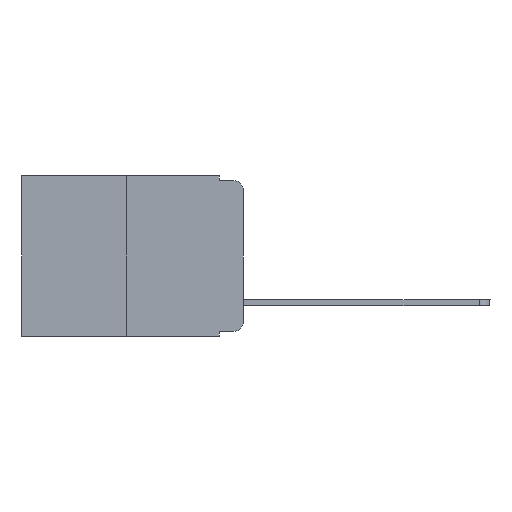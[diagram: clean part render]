
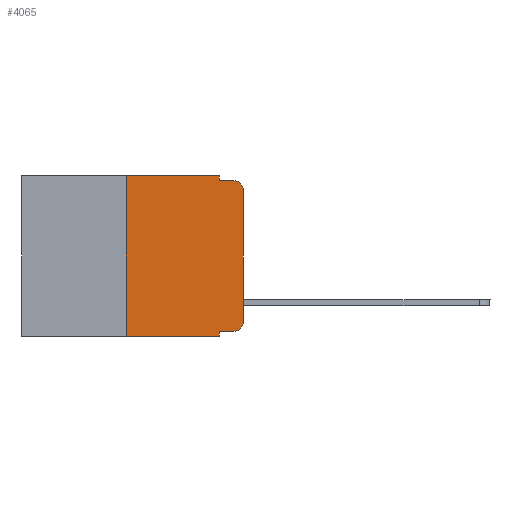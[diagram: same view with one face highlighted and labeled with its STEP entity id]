
A CAD part, left-side view. The second image highlights one B-rep face of the part: STEP entity #4065.
In plain terms, the highlighted planar face has unit normal (-1, 0, 0).
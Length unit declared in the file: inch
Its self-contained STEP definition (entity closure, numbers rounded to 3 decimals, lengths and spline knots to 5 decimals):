
#213 = EDGE_CURVE ( 'NONE', #11336, #13138, #16758, .T. ) ;
#767 = ORIENTED_EDGE ( 'NONE', *, *, #12432, .T. ) ;
#989 = LINE ( 'NONE', #15882, #3333 ) ;
#1069 = EDGE_CURVE ( 'NONE', #6605, #21570, #11862, .T. ) ;
#1149 = ORIENTED_EDGE ( 'NONE', *, *, #22237, .F. ) ;
#1440 = DIRECTION ( 'NONE',  ( 1., 0., 0. ) ) ;
#1817 = EDGE_CURVE ( 'NONE', #21570, #15381, #14677, .T. ) ;
#2532 = CARTESIAN_POINT ( 'NONE',  ( 0., 0.25, 0. ) ) ;
#2564 = VERTEX_POINT ( 'NONE', #3204 ) ;
#2614 = EDGE_CURVE ( 'NONE', #13138, #15381, #2838, .T. ) ;
#2838 = LINE ( 'NONE', #19522, #16950 ) ;
#2845 = DIRECTION ( 'NONE',  ( 0., -1., 0. ) ) ;
#2969 = EDGE_CURVE ( 'NONE', #3411, #2564, #989, .T. ) ;
#3204 = CARTESIAN_POINT ( 'NONE',  ( 0., 0.051, -0.343 ) ) ;
#3275 = CARTESIAN_POINT ( 'NONE',  ( 0., 0., -0.03 ) ) ;
#3333 = VECTOR ( 'NONE', #17605, 39.37008 ) ;
#3411 = VERTEX_POINT ( 'NONE', #10859 ) ;
#3567 = EDGE_LOOP ( 'NONE', ( #13214, #23294, #11967, #9759, #11827, #14202, #8926, #1149, #767, #23444 ) ) ;
#3739 = AXIS2_PLACEMENT_3D ( 'NONE', #19326, #1440, #18484 ) ;
#4037 = EDGE_CURVE ( 'NONE', #23215, #11336, #21836, .T. ) ;
#4065 = ADVANCED_FACE ( 'NONE', ( #21272 ), #13122, .F. ) ;
#5143 = CARTESIAN_POINT ( 'NONE',  ( 0., 0.02, -0.313 ) ) ;
#5422 = VECTOR ( 'NONE', #14570, 39.37008 ) ;
#6605 = VERTEX_POINT ( 'NONE', #20933 ) ;
#6629 = VERTEX_POINT ( 'NONE', #16283 ) ;
#6677 = VECTOR ( 'NONE', #22889, 39.37008 ) ;
#6799 = CARTESIAN_POINT ( 'NONE',  ( 0., 0., 0. ) ) ;
#8610 = AXIS2_PLACEMENT_3D ( 'NONE', #5143, #16107, #12559 ) ;
#8926 = ORIENTED_EDGE ( 'NONE', *, *, #2969, .T. ) ;
#9759 = ORIENTED_EDGE ( 'NONE', *, *, #213, .F. ) ;
#9852 = CIRCLE ( 'NONE', #8610, 0.02 ) ;
#9926 = CARTESIAN_POINT ( 'NONE',  ( 0., 0.051, -0.01 ) ) ;
#10859 = CARTESIAN_POINT ( 'NONE',  ( 0., 0.25, -0.343 ) ) ;
#10968 = LINE ( 'NONE', #19334, #14087 ) ;
#11261 = DIRECTION ( 'NONE',  ( 0., 0., 1. ) ) ;
#11336 = VERTEX_POINT ( 'NONE', #17613 ) ;
#11827 = ORIENTED_EDGE ( 'NONE', *, *, #4037, .F. ) ;
#11862 = LINE ( 'NONE', #6799, #14720 ) ;
#11967 = ORIENTED_EDGE ( 'NONE', *, *, #2614, .F. ) ;
#12007 = VECTOR ( 'NONE', #22891, 39.37008 ) ;
#12027 = CARTESIAN_POINT ( 'NONE',  ( 0., 0.02, -0.03 ) ) ;
#12432 = EDGE_CURVE ( 'NONE', #13806, #6629, #21845, .T. ) ;
#12559 = DIRECTION ( 'NONE',  ( 0., 0., -1. ) ) ;
#12675 = AXIS2_PLACEMENT_3D ( 'NONE', #12027, #14010, #16191 ) ;
#13122 = PLANE ( 'NONE',  #3739 ) ;
#13138 = VERTEX_POINT ( 'NONE', #9926 ) ;
#13214 = ORIENTED_EDGE ( 'NONE', *, *, #1069, .T. ) ;
#13806 = VERTEX_POINT ( 'NONE', #16899 ) ;
#13871 = CARTESIAN_POINT ( 'NONE',  ( 0., 0.473, 0. ) ) ;
#14010 = DIRECTION ( 'NONE',  ( -1., 0., 0. ) ) ;
#14087 = VECTOR ( 'NONE', #11261, 39.37008 ) ;
#14202 = ORIENTED_EDGE ( 'NONE', *, *, #21971, .F. ) ;
#14570 = DIRECTION ( 'NONE',  ( 0., 0., -1. ) ) ;
#14677 = CIRCLE ( 'NONE', #12675, 0.02 ) ;
#14720 = VECTOR ( 'NONE', #21458, 39.37008 ) ;
#15381 = VERTEX_POINT ( 'NONE', #16945 ) ;
#15754 = CARTESIAN_POINT ( 'NONE',  ( 0., 0.051, -0.333 ) ) ;
#15882 = CARTESIAN_POINT ( 'NONE',  ( 0., 0.473, -0.343 ) ) ;
#16107 = DIRECTION ( 'NONE',  ( -1., 0., 0. ) ) ;
#16191 = DIRECTION ( 'NONE',  ( 0., 0., -1. ) ) ;
#16240 = EDGE_CURVE ( 'NONE', #6629, #6605, #9852, .T. ) ;
#16283 = CARTESIAN_POINT ( 'NONE',  ( 0., 0.02, -0.333 ) ) ;
#16758 = LINE ( 'NONE', #23885, #6677 ) ;
#16899 = CARTESIAN_POINT ( 'NONE',  ( 0., 0.051, -0.333 ) ) ;
#16945 = CARTESIAN_POINT ( 'NONE',  ( 0., 0.02, -0.01 ) ) ;
#16950 = VECTOR ( 'NONE', #21392, 39.37008 ) ;
#16955 = LINE ( 'NONE', #21972, #5422 ) ;
#17605 = DIRECTION ( 'NONE',  ( 0., -1., 0. ) ) ;
#17613 = CARTESIAN_POINT ( 'NONE',  ( 0., 0.051, 0. ) ) ;
#18484 = DIRECTION ( 'NONE',  ( 0., 0., -1. ) ) ;
#18655 = VECTOR ( 'NONE', #2845, 39.37008 ) ;
#19326 = CARTESIAN_POINT ( 'NONE',  ( 0., 0.473, 0. ) ) ;
#19334 = CARTESIAN_POINT ( 'NONE',  ( 0., 0.25, 0. ) ) ;
#19522 = CARTESIAN_POINT ( 'NONE',  ( 0., 0.051, -0.01 ) ) ;
#20933 = CARTESIAN_POINT ( 'NONE',  ( 0., 0., -0.313 ) ) ;
#21272 = FACE_OUTER_BOUND ( 'NONE', #3567, .T. ) ;
#21392 = DIRECTION ( 'NONE',  ( 0., -1., 0. ) ) ;
#21458 = DIRECTION ( 'NONE',  ( 0., 0., 1. ) ) ;
#21570 = VERTEX_POINT ( 'NONE', #3275 ) ;
#21836 = LINE ( 'NONE', #13871, #18655 ) ;
#21845 = LINE ( 'NONE', #15754, #12007 ) ;
#21971 = EDGE_CURVE ( 'NONE', #3411, #23215, #10968, .T. ) ;
#21972 = CARTESIAN_POINT ( 'NONE',  ( 0., 0.051, 0. ) ) ;
#22237 = EDGE_CURVE ( 'NONE', #13806, #2564, #16955, .T. ) ;
#22889 = DIRECTION ( 'NONE',  ( 0., 0., -1. ) ) ;
#22891 = DIRECTION ( 'NONE',  ( 0., -1., 0. ) ) ;
#23215 = VERTEX_POINT ( 'NONE', #2532 ) ;
#23294 = ORIENTED_EDGE ( 'NONE', *, *, #1817, .T. ) ;
#23444 = ORIENTED_EDGE ( 'NONE', *, *, #16240, .T. ) ;
#23885 = CARTESIAN_POINT ( 'NONE',  ( 0., 0.051, 0. ) ) ;
